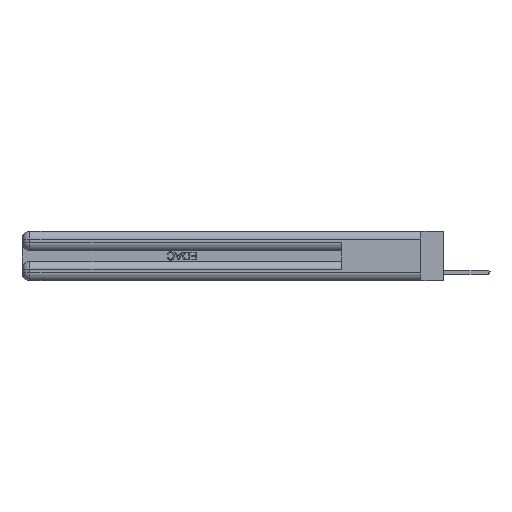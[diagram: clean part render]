
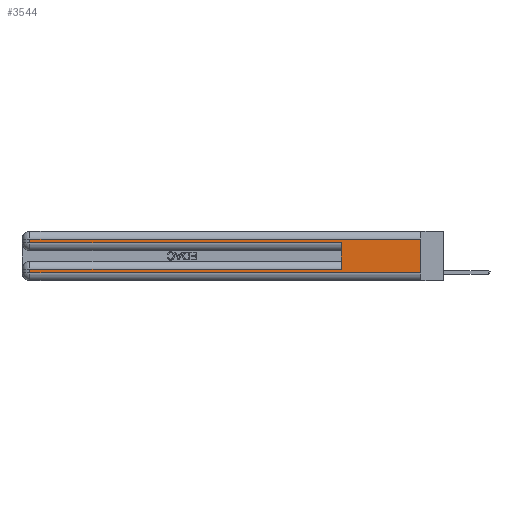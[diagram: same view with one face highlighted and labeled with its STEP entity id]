
A CAD part, left-side view. The second image highlights one B-rep face of the part: STEP entity #3544.
In plain terms, the highlighted planar face has unit normal (-1, 0, 0).
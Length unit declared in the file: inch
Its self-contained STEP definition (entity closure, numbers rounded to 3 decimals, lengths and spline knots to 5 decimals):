
#162 = AXIS2_PLACEMENT_3D ( 'NONE', #20801, #8841, #13938 ) ;
#196 = EDGE_CURVE ( 'NONE', #21278, #27774, #23379, .T. ) ;
#841 = VECTOR ( 'NONE', #20828, 39.37008 ) ;
#860 = FACE_OUTER_BOUND ( 'NONE', #10195, .T. ) ;
#983 = DIRECTION ( 'NONE',  ( 0., 1., 0. ) ) ;
#1529 = VECTOR ( 'NONE', #983, 39.37008 ) ;
#3516 = ORIENTED_EDGE ( 'NONE', *, *, #17277, .T. ) ;
#3544 = ADVANCED_FACE ( 'NONE', ( #860 ), #10815, .F. ) ;
#3577 = ORIENTED_EDGE ( 'NONE', *, *, #26717, .T. ) ;
#3645 = LINE ( 'NONE', #3972, #841 ) ;
#3854 = DIRECTION ( 'NONE',  ( 0., 0., -1. ) ) ;
#3972 = CARTESIAN_POINT ( 'NONE',  ( 0., 0., 0.31 ) ) ;
#4240 = CARTESIAN_POINT ( 'NONE',  ( 0., 2.94, 0.37 ) ) ;
#4253 = VECTOR ( 'NONE', #26807, 39.37008 ) ;
#5779 = VECTOR ( 'NONE', #3854, 39.37008 ) ;
#6061 = CARTESIAN_POINT ( 'NONE',  ( 0., 0., 0.31 ) ) ;
#6140 = CARTESIAN_POINT ( 'NONE',  ( 0., 2.94, 0.37 ) ) ;
#6836 = LINE ( 'NONE', #4240, #4253 ) ;
#6933 = EDGE_CURVE ( 'NONE', #15859, #30371, #9026, .T. ) ;
#8034 = EDGE_CURVE ( 'NONE', #15859, #9205, #3645, .T. ) ;
#8262 = DIRECTION ( 'NONE',  ( 0., -1., 0. ) ) ;
#8841 = DIRECTION ( 'NONE',  ( 1., 0., 0. ) ) ;
#8918 = CARTESIAN_POINT ( 'NONE',  ( 0., 0., 0.285 ) ) ;
#9026 = LINE ( 'NONE', #28831, #23970 ) ;
#9205 = VERTEX_POINT ( 'NONE', #27586 ) ;
#9976 = VERTEX_POINT ( 'NONE', #11913 ) ;
#10195 = EDGE_LOOP ( 'NONE', ( #19152, #19423, #3577, #16807, #24441, #17218, #13255, #3516 ) ) ;
#10815 = PLANE ( 'NONE',  #162 ) ;
#11022 = LINE ( 'NONE', #31311, #19194 ) ;
#11732 = VECTOR ( 'NONE', #11917, 39.37008 ) ;
#11913 = CARTESIAN_POINT ( 'NONE',  ( 0., 2.94, 0.285 ) ) ;
#11917 = DIRECTION ( 'NONE',  ( 0., 0., 1. ) ) ;
#12397 = LINE ( 'NONE', #22389, #11732 ) ;
#13255 = ORIENTED_EDGE ( 'NONE', *, *, #22474, .T. ) ;
#13792 = CARTESIAN_POINT ( 'NONE',  ( 0., 0.6, 0.285 ) ) ;
#13938 = DIRECTION ( 'NONE',  ( 0., 0., -1. ) ) ;
#14002 = LINE ( 'NONE', #6140, #5779 ) ;
#15250 = VERTEX_POINT ( 'NONE', #28581 ) ;
#15344 = CARTESIAN_POINT ( 'NONE',  ( 0., 2.94, 0.085 ) ) ;
#15859 = VERTEX_POINT ( 'NONE', #6061 ) ;
#16807 = ORIENTED_EDGE ( 'NONE', *, *, #29422, .T. ) ;
#17218 = ORIENTED_EDGE ( 'NONE', *, *, #196, .T. ) ;
#17277 = EDGE_CURVE ( 'NONE', #15250, #30371, #11022, .T. ) ;
#18261 = LINE ( 'NONE', #8918, #29973 ) ;
#18388 = DIRECTION ( 'NONE',  ( 0., -1., 0. ) ) ;
#18640 = CARTESIAN_POINT ( 'NONE',  ( 0., 0., 0.085 ) ) ;
#19031 = DIRECTION ( 'NONE',  ( 0., 0., -1. ) ) ;
#19152 = ORIENTED_EDGE ( 'NONE', *, *, #6933, .F. ) ;
#19194 = VECTOR ( 'NONE', #18388, 39.37008 ) ;
#19423 = ORIENTED_EDGE ( 'NONE', *, *, #8034, .T. ) ;
#20801 = CARTESIAN_POINT ( 'NONE',  ( 0., 0., 0.37 ) ) ;
#20828 = DIRECTION ( 'NONE',  ( 0., 1., 0. ) ) ;
#21278 = VERTEX_POINT ( 'NONE', #29114 ) ;
#21935 = CARTESIAN_POINT ( 'NONE',  ( 0., 0., 0.06 ) ) ;
#22389 = CARTESIAN_POINT ( 'NONE',  ( 0., 0.6, 0.145 ) ) ;
#22474 = EDGE_CURVE ( 'NONE', #27774, #15250, #6836, .T. ) ;
#23379 = LINE ( 'NONE', #18640, #1529 ) ;
#23970 = VECTOR ( 'NONE', #19031, 39.37008 ) ;
#24441 = ORIENTED_EDGE ( 'NONE', *, *, #32314, .F. ) ;
#25602 = VERTEX_POINT ( 'NONE', #13792 ) ;
#26717 = EDGE_CURVE ( 'NONE', #9205, #9976, #14002, .T. ) ;
#26807 = DIRECTION ( 'NONE',  ( 0., 0., -1. ) ) ;
#27586 = CARTESIAN_POINT ( 'NONE',  ( 0., 2.94, 0.31 ) ) ;
#27774 = VERTEX_POINT ( 'NONE', #15344 ) ;
#28581 = CARTESIAN_POINT ( 'NONE',  ( 0., 2.94, 0.06 ) ) ;
#28831 = CARTESIAN_POINT ( 'NONE',  ( 0., 0., 0.37 ) ) ;
#29114 = CARTESIAN_POINT ( 'NONE',  ( 0., 0.6, 0.085 ) ) ;
#29422 = EDGE_CURVE ( 'NONE', #9976, #25602, #18261, .T. ) ;
#29973 = VECTOR ( 'NONE', #8262, 39.37008 ) ;
#30371 = VERTEX_POINT ( 'NONE', #21935 ) ;
#31311 = CARTESIAN_POINT ( 'NONE',  ( 0., 0., 0.06 ) ) ;
#32314 = EDGE_CURVE ( 'NONE', #21278, #25602, #12397, .T. ) ;
